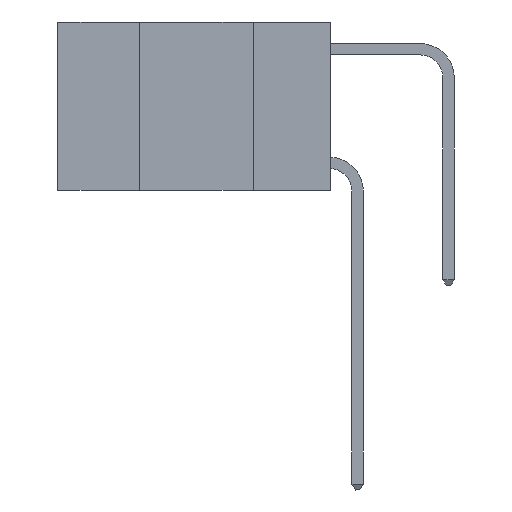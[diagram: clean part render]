
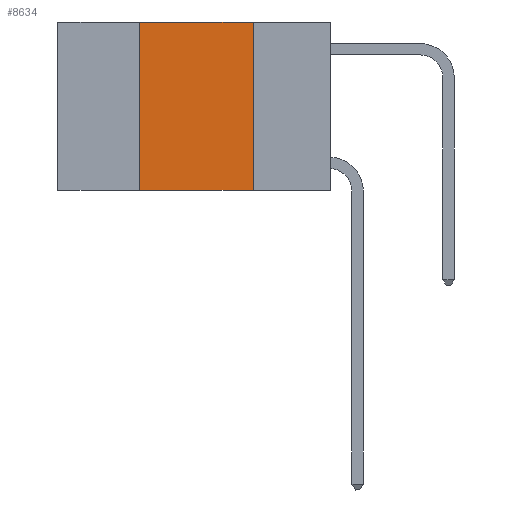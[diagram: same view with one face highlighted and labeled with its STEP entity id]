
A CAD part, left-side view. The second image highlights one B-rep face of the part: STEP entity #8634.
In plain terms, the highlighted planar face has unit normal (-1, 0, 0).
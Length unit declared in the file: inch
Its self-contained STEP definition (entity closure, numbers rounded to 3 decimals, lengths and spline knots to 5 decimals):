
#779 = CARTESIAN_POINT ( 'NONE',  ( 0., 0.42, 0. ) ) ;
#1176 = VERTEX_POINT ( 'NONE', #4631 ) ;
#1325 = VECTOR ( 'NONE', #11967, 39.37008 ) ;
#1770 = AXIS2_PLACEMENT_3D ( 'NONE', #14554, #20795, #11413 ) ;
#1933 = CARTESIAN_POINT ( 'NONE',  ( 0., 0.17, -0.37 ) ) ;
#2174 = EDGE_CURVE ( 'NONE', #1176, #4282, #5313, .T. ) ;
#2286 = LINE ( 'NONE', #4949, #19105 ) ;
#4282 = VERTEX_POINT ( 'NONE', #1933 ) ;
#4631 = CARTESIAN_POINT ( 'NONE',  ( 0., 0.42, -0.37 ) ) ;
#4708 = PLANE ( 'NONE',  #1770 ) ;
#4780 = DIRECTION ( 'NONE',  ( 0., -1., 0. ) ) ;
#4949 = CARTESIAN_POINT ( 'NONE',  ( 0., 0.42, 0. ) ) ;
#5313 = LINE ( 'NONE', #16478, #1325 ) ;
#5782 = LINE ( 'NONE', #9491, #19146 ) ;
#5803 = ORIENTED_EDGE ( 'NONE', *, *, #8646, .F. ) ;
#7470 = EDGE_CURVE ( 'NONE', #15560, #4282, #5782, .T. ) ;
#8265 = EDGE_CURVE ( 'NONE', #1176, #13161, #2286, .T. ) ;
#8634 = ADVANCED_FACE ( 'NONE', ( #15708 ), #4708, .F. ) ;
#8646 = EDGE_CURVE ( 'NONE', #13161, #15560, #10957, .T. ) ;
#9491 = CARTESIAN_POINT ( 'NONE',  ( 0., 0.17, 0. ) ) ;
#9580 = EDGE_LOOP ( 'NONE', ( #19537, #5803, #11638, #10252 ) ) ;
#10252 = ORIENTED_EDGE ( 'NONE', *, *, #2174, .T. ) ;
#10957 = LINE ( 'NONE', #13022, #19362 ) ;
#11413 = DIRECTION ( 'NONE',  ( 0., 0., -1. ) ) ;
#11633 = DIRECTION ( 'NONE',  ( 0., 0., 1. ) ) ;
#11638 = ORIENTED_EDGE ( 'NONE', *, *, #8265, .F. ) ;
#11967 = DIRECTION ( 'NONE',  ( 0., -1., 0. ) ) ;
#13022 = CARTESIAN_POINT ( 'NONE',  ( 0., 0.6, 0. ) ) ;
#13161 = VERTEX_POINT ( 'NONE', #779 ) ;
#14052 = CARTESIAN_POINT ( 'NONE',  ( 0., 0.17, 0. ) ) ;
#14554 = CARTESIAN_POINT ( 'NONE',  ( 0., 0.6, 0. ) ) ;
#15560 = VERTEX_POINT ( 'NONE', #14052 ) ;
#15708 = FACE_OUTER_BOUND ( 'NONE', #9580, .T. ) ;
#16478 = CARTESIAN_POINT ( 'NONE',  ( 0., 0.6, -0.37 ) ) ;
#18984 = DIRECTION ( 'NONE',  ( 0., 0., -1. ) ) ;
#19105 = VECTOR ( 'NONE', #11633, 39.37008 ) ;
#19146 = VECTOR ( 'NONE', #18984, 39.37008 ) ;
#19362 = VECTOR ( 'NONE', #4780, 39.37008 ) ;
#19537 = ORIENTED_EDGE ( 'NONE', *, *, #7470, .F. ) ;
#20795 = DIRECTION ( 'NONE',  ( 1., 0., 0. ) ) ;
